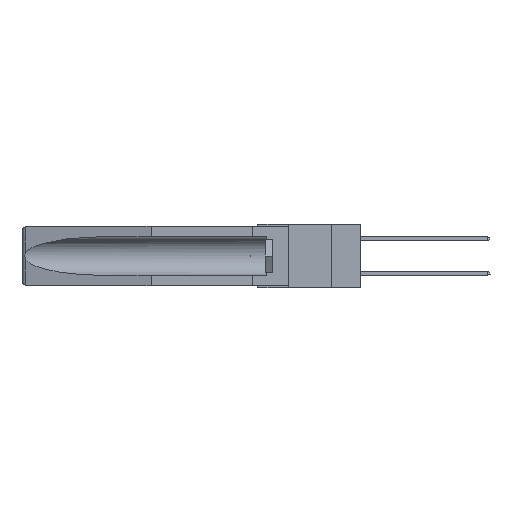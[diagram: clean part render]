
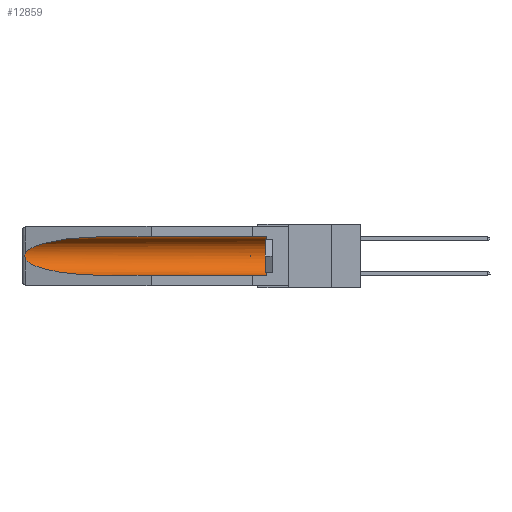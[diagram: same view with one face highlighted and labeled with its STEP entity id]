
A CAD part, left-side view. The second image highlights one B-rep face of the part: STEP entity #12859.
In plain terms, the highlighted cylindrical face has radius 2.857 mm (diameter 5.715 mm), a partial arc.
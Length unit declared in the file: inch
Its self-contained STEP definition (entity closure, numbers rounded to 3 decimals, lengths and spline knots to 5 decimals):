
#1099 = EDGE_CURVE ( 'NONE', #6195, #33924, #16475, .T. ) ;
#1835 = CARTESIAN_POINT ( 'NONE',  ( 0.2673, 1.53269, -0.17917 ) ) ;
#2057 = CARTESIAN_POINT ( 'NONE',  ( 0.25451, 1.48313, -0.24835 ) ) ;
#2058 = CARTESIAN_POINT ( 'NONE',  ( 0.155, 0.126, -0.059 ) ) ;
#2279 = CARTESIAN_POINT ( 'NONE',  ( 0.26537, 1.52718, -0.19328 ) ) ;
#2418 = CARTESIAN_POINT ( 'NONE',  ( 0.155, -0.30754, -0.284 ) ) ;
#2546 = EDGE_CURVE ( 'NONE', #7369, #9171, #34442, .T. ) ;
#3288 = DIRECTION ( 'NONE',  ( 0., 1., 0. ) ) ;
#4420 = CARTESIAN_POINT ( 'NONE',  ( 0.26537, 1.52718, -0.14972 ) ) ;
#4750 =( BOUNDED_CURVE ( )  B_SPLINE_CURVE ( 3, ( #9920, #31542, #34001, #17688 ),
 .UNSPECIFIED., .F., .F. ) 
 B_SPLINE_CURVE_WITH_KNOTS ( ( 4, 4 ),
 ( 4.71239, 6.08839 ),
 .UNSPECIFIED. ) 
 CURVE ( )  GEOMETRIC_REPRESENTATION_ITEM ( )  RATIONAL_B_SPLINE_CURVE ( ( 1., 0.848, 0.848, 1. ) ) 
 REPRESENTATION_ITEM ( '' )  );
#6099 = CARTESIAN_POINT ( 'NONE',  ( 0.155, 0.126, -0.284 ) ) ;
#6195 = VERTEX_POINT ( 'NONE', #6099 ) ;
#6765 = VECTOR ( 'NONE', #7874, 39.37008 ) ;
#6968 = ORIENTED_EDGE ( 'NONE', *, *, #20704, .T. ) ;
#7005 = AXIS2_PLACEMENT_3D ( 'NONE', #17051, #30457, #19415 ) ;
#7031 = CARTESIAN_POINT ( 'NONE',  ( 0.26655, 1.53094, -0.18657 ) ) ;
#7153 = CARTESIAN_POINT ( 'NONE',  ( 0.26537, 1.52718, -0.19328 ) ) ;
#7369 = VERTEX_POINT ( 'NONE', #14366 ) ;
#7874 = DIRECTION ( 'NONE',  ( 0., 1., 0. ) ) ;
#9171 = VERTEX_POINT ( 'NONE', #2279 ) ;
#9642 = LINE ( 'NONE', #11230, #17658 ) ;
#9920 = CARTESIAN_POINT ( 'NONE',  ( 0.155, 1.07973, -0.059 ) ) ;
#11230 = CARTESIAN_POINT ( 'NONE',  ( 0.155, -0.30754, -0.059 ) ) ;
#12145 = CARTESIAN_POINT ( 'NONE',  ( 0.155, 1.07973, -0.284 ) ) ;
#12856 = CIRCLE ( 'NONE', #7005, 0.1125 ) ;
#12859 = ADVANCED_FACE ( 'NONE', ( #31085 ), #27719, .F. ) ;
#13351 = EDGE_CURVE ( 'NONE', #18924, #7369, #4750, .T. ) ;
#13732 = ORIENTED_EDGE ( 'NONE', *, *, #15117, .T. ) ;
#14252 = ORIENTED_EDGE ( 'NONE', *, *, #14559, .T. ) ;
#14366 = CARTESIAN_POINT ( 'NONE',  ( 0.26537, 1.52718, -0.14972 ) ) ;
#14559 = EDGE_CURVE ( 'NONE', #6195, #25427, #12856, .T. ) ;
#15117 = EDGE_CURVE ( 'NONE', #9171, #33924, #24281, .T. ) ;
#15391 = CARTESIAN_POINT ( 'NONE',  ( 0.21114, 1.30732, -0.284 ) ) ;
#15835 = EDGE_LOOP ( 'NONE', ( #16002, #23516, #13732, #27297, #14252, #6968 ) ) ;
#16002 = ORIENTED_EDGE ( 'NONE', *, *, #13351, .T. ) ;
#16475 = LINE ( 'NONE', #2418, #6765 ) ;
#17051 = CARTESIAN_POINT ( 'NONE',  ( 0.155, 0.126, -0.1715 ) ) ;
#17658 = VECTOR ( 'NONE', #3288, 39.37008 ) ;
#17688 = CARTESIAN_POINT ( 'NONE',  ( 0.26537, 1.52718, -0.14972 ) ) ;
#17775 = CARTESIAN_POINT ( 'NONE',  ( 0.2673, 1.5327, -0.16383 ) ) ;
#18051 = AXIS2_PLACEMENT_3D ( 'NONE', #20920, #34607, #29793 ) ;
#18102 = CARTESIAN_POINT ( 'NONE',  ( 0.26537, 1.52718, -0.19328 ) ) ;
#18924 = VERTEX_POINT ( 'NONE', #28159 ) ;
#19415 = DIRECTION ( 'NONE',  ( 0., 0., 1. ) ) ;
#20499 = CARTESIAN_POINT ( 'NONE',  ( 0.2675, 1.53308, -0.16763 ) ) ;
#20704 = EDGE_CURVE ( 'NONE', #25427, #18924, #9642, .T. ) ;
#20920 = CARTESIAN_POINT ( 'NONE',  ( 0.155, -0.30754, -0.1715 ) ) ;
#23220 = CARTESIAN_POINT ( 'NONE',  ( 0.2675, 1.53308, -0.17534 ) ) ;
#23516 = ORIENTED_EDGE ( 'NONE', *, *, #2546, .T. ) ;
#24281 =( BOUNDED_CURVE ( )  B_SPLINE_CURVE ( 3, ( #7153, #2057, #15391, #26105 ),
 .UNSPECIFIED., .F., .F. ) 
 B_SPLINE_CURVE_WITH_KNOTS ( ( 4, 4 ),
 ( 0.1948, 1.5708 ),
 .UNSPECIFIED. ) 
 CURVE ( )  GEOMETRIC_REPRESENTATION_ITEM ( )  RATIONAL_B_SPLINE_CURVE ( ( 1., 0.848, 0.848, 1. ) ) 
 REPRESENTATION_ITEM ( '' )  );
#25427 = VERTEX_POINT ( 'NONE', #2058 ) ;
#25869 = CARTESIAN_POINT ( 'NONE',  ( 0.26654, 1.53092, -0.15636 ) ) ;
#26090 = CARTESIAN_POINT ( 'NONE',  ( 0.26597, 1.5296, -0.19026 ) ) ;
#26105 = CARTESIAN_POINT ( 'NONE',  ( 0.155, 1.07973, -0.284 ) ) ;
#27297 = ORIENTED_EDGE ( 'NONE', *, *, #1099, .F. ) ;
#27719 = CYLINDRICAL_SURFACE ( 'NONE', #18051, 0.1125 ) ;
#28159 = CARTESIAN_POINT ( 'NONE',  ( 0.155, 1.07973, -0.059 ) ) ;
#29793 = DIRECTION ( 'NONE',  ( 0., 0., 1. ) ) ;
#30457 = DIRECTION ( 'NONE',  ( 0., -1., 0. ) ) ;
#31085 = FACE_OUTER_BOUND ( 'NONE', #15835, .T. ) ;
#31542 = CARTESIAN_POINT ( 'NONE',  ( 0.21114, 1.30732, -0.059 ) ) ;
#33924 = VERTEX_POINT ( 'NONE', #12145 ) ;
#34001 = CARTESIAN_POINT ( 'NONE',  ( 0.25451, 1.48313, -0.09465 ) ) ;
#34442 = B_SPLINE_CURVE_WITH_KNOTS ( 'NONE', 3,
 ( #4420, #34441, #25869, #17775, #20499, #23220, #1835, #7031, #26090, #18102 ),
 .UNSPECIFIED., .F., .F.,
 ( 4, 2, 2, 2, 4 ),
 ( 0., 0.00029, 0.00058, 0.00087, 0.00117 ),
 .UNSPECIFIED. ) ;
#34441 = CARTESIAN_POINT ( 'NONE',  ( 0.26597, 1.52961, -0.15275 ) ) ;
#34607 = DIRECTION ( 'NONE',  ( 0., 1., 0. ) ) ;
